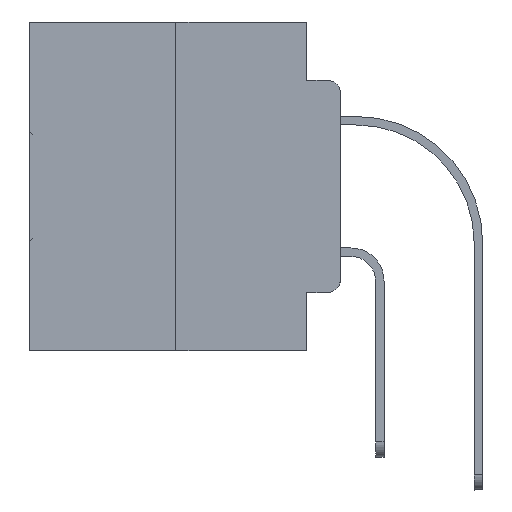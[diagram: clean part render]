
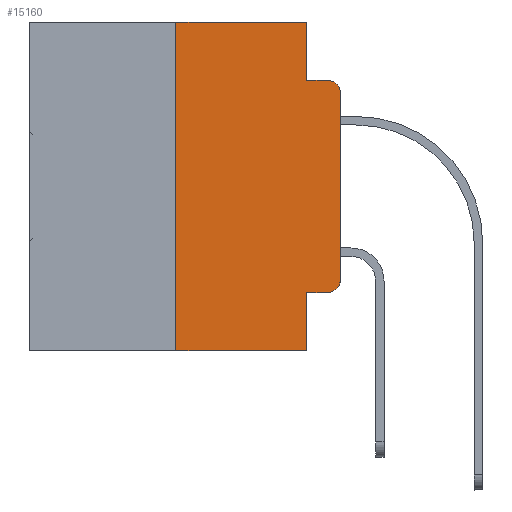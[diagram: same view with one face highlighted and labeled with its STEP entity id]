
A CAD part, left-side view. The second image highlights one B-rep face of the part: STEP entity #15160.
In plain terms, the highlighted planar face has unit normal (-1, 0, 0).
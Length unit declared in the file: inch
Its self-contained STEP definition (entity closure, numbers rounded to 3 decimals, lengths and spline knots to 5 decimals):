
#10 = EDGE_CURVE ( 'NONE', #23920, #32545, #22324, .T. ) ;
#260 = ORIENTED_EDGE ( 'NONE', *, *, #23057, .T. ) ;
#708 = CARTESIAN_POINT ( 'NONE',  ( 0., 0.051, -0.4115 ) ) ;
#758 = VERTEX_POINT ( 'NONE', #10806 ) ;
#896 = EDGE_CURVE ( 'NONE', #19178, #23920, #7253, .T. ) ;
#1493 = LINE ( 'NONE', #4228, #16184 ) ;
#1708 = LINE ( 'NONE', #30158, #20151 ) ;
#2109 = VECTOR ( 'NONE', #22037, 39.37008 ) ;
#2555 = DIRECTION ( 'NONE',  ( -1., 0., 0. ) ) ;
#2900 = DIRECTION ( 'NONE',  ( 0., 0., -1. ) ) ;
#2949 = VECTOR ( 'NONE', #22632, 39.37008 ) ;
#3182 = VERTEX_POINT ( 'NONE', #10467 ) ;
#4155 = DIRECTION ( 'NONE',  ( 0., 0., 1. ) ) ;
#4198 = VECTOR ( 'NONE', #9985, 39.37008 ) ;
#4228 = CARTESIAN_POINT ( 'NONE',  ( 0., 0.473, -0.5 ) ) ;
#4287 = DIRECTION ( 'NONE',  ( 0., 0., -1. ) ) ;
#4339 = EDGE_CURVE ( 'NONE', #758, #12047, #22630, .T. ) ;
#4388 = CARTESIAN_POINT ( 'NONE',  ( 0., 0.473, 0. ) ) ;
#4565 = DIRECTION ( 'NONE',  ( 1., 0., 0. ) ) ;
#4983 = ORIENTED_EDGE ( 'NONE', *, *, #28305, .F. ) ;
#5926 = EDGE_CURVE ( 'NONE', #17223, #11384, #19516, .T. ) ;
#6705 = DIRECTION ( 'NONE',  ( 0., -1., 0. ) ) ;
#6977 = CARTESIAN_POINT ( 'NONE',  ( 0., 0.02, -0.3915 ) ) ;
#7253 = CIRCLE ( 'NONE', #21375, 0.02 ) ;
#7315 = ORIENTED_EDGE ( 'NONE', *, *, #4339, .F. ) ;
#9578 = DIRECTION ( 'NONE',  ( 0., -1., 0. ) ) ;
#9626 = CARTESIAN_POINT ( 'NONE',  ( 0., 0.051, -0.0885 ) ) ;
#9985 = DIRECTION ( 'NONE',  ( 0., -1., 0. ) ) ;
#10467 = CARTESIAN_POINT ( 'NONE',  ( 0., 0.02, -0.0885 ) ) ;
#10806 = CARTESIAN_POINT ( 'NONE',  ( 0., 0.051, 0. ) ) ;
#10864 = EDGE_CURVE ( 'NONE', #28095, #11384, #1493, .T. ) ;
#11384 = VERTEX_POINT ( 'NONE', #18107 ) ;
#12047 = VERTEX_POINT ( 'NONE', #33718 ) ;
#12278 = DIRECTION ( 'NONE',  ( -1., 0., 0. ) ) ;
#12735 = ORIENTED_EDGE ( 'NONE', *, *, #10, .T. ) ;
#12965 = LINE ( 'NONE', #23405, #2109 ) ;
#13874 = AXIS2_PLACEMENT_3D ( 'NONE', #31012, #2555, #2900 ) ;
#14669 = PLANE ( 'NONE',  #26362 ) ;
#15106 = CARTESIAN_POINT ( 'NONE',  ( 0., 0.473, 0. ) ) ;
#15160 = ADVANCED_FACE ( 'NONE', ( #17412 ), #14669, .F. ) ;
#15573 = CARTESIAN_POINT ( 'NONE',  ( 0., 0.02, -0.4115 ) ) ;
#16184 = VECTOR ( 'NONE', #9578, 39.37008 ) ;
#16489 = ORIENTED_EDGE ( 'NONE', *, *, #10864, .T. ) ;
#17059 = ORIENTED_EDGE ( 'NONE', *, *, #19828, .T. ) ;
#17140 = VERTEX_POINT ( 'NONE', #18554 ) ;
#17223 = VERTEX_POINT ( 'NONE', #708 ) ;
#17318 = CARTESIAN_POINT ( 'NONE',  ( 0., 0.051, 0. ) ) ;
#17412 = FACE_OUTER_BOUND ( 'NONE', #28706, .T. ) ;
#18107 = CARTESIAN_POINT ( 'NONE',  ( 0., 0.051, -0.5 ) ) ;
#18548 = CARTESIAN_POINT ( 'NONE',  ( 0., 0.25, -0.5 ) ) ;
#18554 = CARTESIAN_POINT ( 'NONE',  ( 0., 0.25, 0. ) ) ;
#19178 = VERTEX_POINT ( 'NONE', #15573 ) ;
#19516 = LINE ( 'NONE', #22093, #29947 ) ;
#19558 = CARTESIAN_POINT ( 'NONE',  ( 0., 0., -0.3915 ) ) ;
#19688 = DIRECTION ( 'NONE',  ( 0., 0., -1. ) ) ;
#19775 = CARTESIAN_POINT ( 'NONE',  ( 0., 0., 0. ) ) ;
#19828 = EDGE_CURVE ( 'NONE', #17223, #19178, #1708, .T. ) ;
#20151 = VECTOR ( 'NONE', #6705, 39.37008 ) ;
#20531 = EDGE_CURVE ( 'NONE', #28095, #17140, #12965, .T. ) ;
#21133 = ORIENTED_EDGE ( 'NONE', *, *, #24007, .F. ) ;
#21375 = AXIS2_PLACEMENT_3D ( 'NONE', #6977, #12278, #32333 ) ;
#22037 = DIRECTION ( 'NONE',  ( 0., 0., 1. ) ) ;
#22093 = CARTESIAN_POINT ( 'NONE',  ( 0., 0.051, 0. ) ) ;
#22324 = LINE ( 'NONE', #19775, #22985 ) ;
#22630 = LINE ( 'NONE', #17318, #23434 ) ;
#22632 = DIRECTION ( 'NONE',  ( 0., -1., 0. ) ) ;
#22726 = DIRECTION ( 'NONE',  ( 0., 0., -1. ) ) ;
#22866 = CARTESIAN_POINT ( 'NONE',  ( 0., 0., -0.1085 ) ) ;
#22985 = VECTOR ( 'NONE', #4155, 39.37008 ) ;
#23057 = EDGE_CURVE ( 'NONE', #32545, #3182, #28634, .T. ) ;
#23405 = CARTESIAN_POINT ( 'NONE',  ( 0., 0.25, 0. ) ) ;
#23434 = VECTOR ( 'NONE', #4287, 39.37008 ) ;
#23920 = VERTEX_POINT ( 'NONE', #19558 ) ;
#24007 = EDGE_CURVE ( 'NONE', #12047, #3182, #26170, .T. ) ;
#25566 = ORIENTED_EDGE ( 'NONE', *, *, #20531, .F. ) ;
#26170 = LINE ( 'NONE', #9626, #2949 ) ;
#26362 = AXIS2_PLACEMENT_3D ( 'NONE', #4388, #4565, #22726 ) ;
#27544 = ORIENTED_EDGE ( 'NONE', *, *, #896, .T. ) ;
#28095 = VERTEX_POINT ( 'NONE', #18548 ) ;
#28305 = EDGE_CURVE ( 'NONE', #17140, #758, #30182, .T. ) ;
#28634 = CIRCLE ( 'NONE', #13874, 0.02 ) ;
#28706 = EDGE_LOOP ( 'NONE', ( #12735, #260, #21133, #7315, #4983, #25566, #16489, #31589, #17059, #27544 ) ) ;
#29947 = VECTOR ( 'NONE', #19688, 39.37008 ) ;
#30158 = CARTESIAN_POINT ( 'NONE',  ( 0., 0.051, -0.4115 ) ) ;
#30182 = LINE ( 'NONE', #15106, #4198 ) ;
#31012 = CARTESIAN_POINT ( 'NONE',  ( 0., 0.02, -0.1085 ) ) ;
#31589 = ORIENTED_EDGE ( 'NONE', *, *, #5926, .F. ) ;
#32333 = DIRECTION ( 'NONE',  ( 0., 0., -1. ) ) ;
#32545 = VERTEX_POINT ( 'NONE', #22866 ) ;
#33718 = CARTESIAN_POINT ( 'NONE',  ( 0., 0.051, -0.0885 ) ) ;
